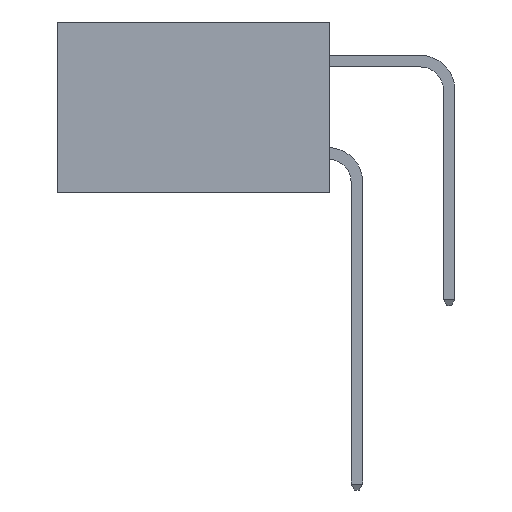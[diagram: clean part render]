
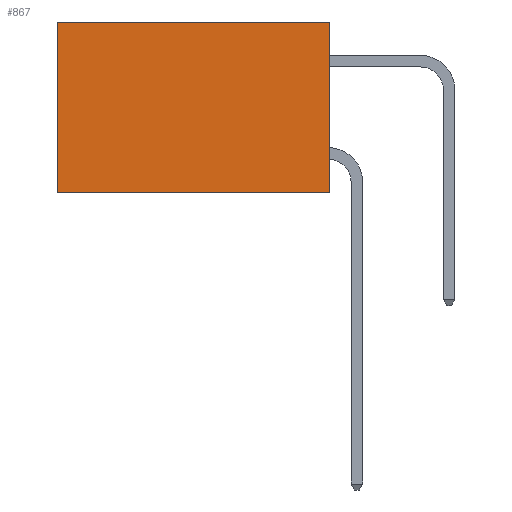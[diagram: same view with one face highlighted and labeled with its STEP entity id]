
A CAD part, left-side view. The second image highlights one B-rep face of the part: STEP entity #867.
In plain terms, the highlighted planar face has unit normal (-1, 0, 0).
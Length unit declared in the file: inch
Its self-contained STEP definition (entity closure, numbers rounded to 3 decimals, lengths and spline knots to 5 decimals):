
#849 = CARTESIAN_POINT ( 'NONE',  ( 0.277, 0.59, 0. ) ) ;
#867 = ADVANCED_FACE ( 'NONE', ( #6453 ), #3738, .F. ) ;
#1040 = ORIENTED_EDGE ( 'NONE', *, *, #3574, .T. ) ;
#1076 = ORIENTED_EDGE ( 'NONE', *, *, #5365, .F. ) ;
#1085 = ORIENTED_EDGE ( 'NONE', *, *, #7897, .F. ) ;
#1131 = ORIENTED_EDGE ( 'NONE', *, *, #8800, .T. ) ;
#1722 = LINE ( 'NONE', #8303, #7473 ) ;
#1766 = LINE ( 'NONE', #6489, #7508 ) ;
#1879 = VERTEX_POINT ( 'NONE', #8666 ) ;
#2881 = VERTEX_POINT ( 'NONE', #3534 ) ;
#2900 = DIRECTION ( 'NONE',  ( 0., 0., -1. ) ) ;
#3534 = CARTESIAN_POINT ( 'NONE',  ( 0.277, 0.59, -0.37 ) ) ;
#3574 = EDGE_CURVE ( 'NONE', #6232, #2881, #1766, .T. ) ;
#3738 = PLANE ( 'NONE',  #7462 ) ;
#3918 = LINE ( 'NONE', #4551, #5321 ) ;
#4551 = CARTESIAN_POINT ( 'NONE',  ( 0.277, 0., 0. ) ) ;
#5321 = VECTOR ( 'NONE', #6927, 39.37008 ) ;
#5365 = EDGE_CURVE ( 'NONE', #8317, #2881, #1722, .T. ) ;
#6043 = VECTOR ( 'NONE', #2900, 39.37008 ) ;
#6232 = VERTEX_POINT ( 'NONE', #849 ) ;
#6445 = DIRECTION ( 'NONE',  ( 0., 0., -1. ) ) ;
#6453 = FACE_OUTER_BOUND ( 'NONE', #8912, .T. ) ;
#6489 = CARTESIAN_POINT ( 'NONE',  ( 0.277, 0.59, -0.37 ) ) ;
#6545 = CARTESIAN_POINT ( 'NONE',  ( 0.277, 0., -0.37 ) ) ;
#6927 = DIRECTION ( 'NONE',  ( 0., 1., 0. ) ) ;
#7050 = DIRECTION ( 'NONE',  ( 1., 0., 0. ) ) ;
#7462 = AXIS2_PLACEMENT_3D ( 'NONE', #9656, #7050, #7642 ) ;
#7473 = VECTOR ( 'NONE', #9652, 39.37008 ) ;
#7508 = VECTOR ( 'NONE', #6445, 39.37008 ) ;
#7642 = DIRECTION ( 'NONE',  ( 0., 0., -1. ) ) ;
#7897 = EDGE_CURVE ( 'NONE', #1879, #8317, #9791, .T. ) ;
#8190 = CARTESIAN_POINT ( 'NONE',  ( 0.277, 0., -0.37 ) ) ;
#8303 = CARTESIAN_POINT ( 'NONE',  ( 0.277, 0., -0.37 ) ) ;
#8317 = VERTEX_POINT ( 'NONE', #6545 ) ;
#8666 = CARTESIAN_POINT ( 'NONE',  ( 0.277, 0., 0. ) ) ;
#8800 = EDGE_CURVE ( 'NONE', #1879, #6232, #3918, .T. ) ;
#8912 = EDGE_LOOP ( 'NONE', ( #1040, #1076, #1085, #1131 ) ) ;
#9652 = DIRECTION ( 'NONE',  ( 0., 1., 0. ) ) ;
#9656 = CARTESIAN_POINT ( 'NONE',  ( 0.277, 0., -0.37 ) ) ;
#9791 = LINE ( 'NONE', #8190, #6043 ) ;
